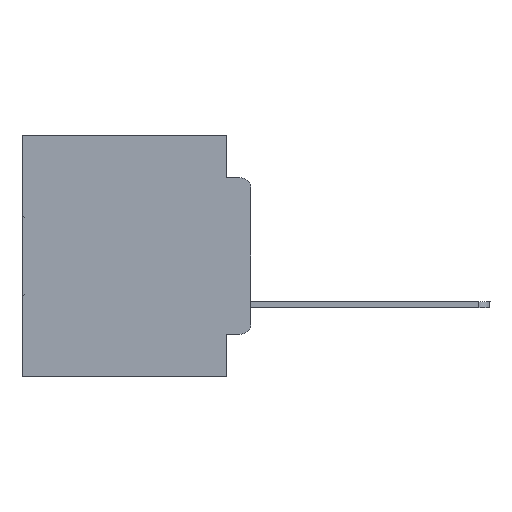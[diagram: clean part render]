
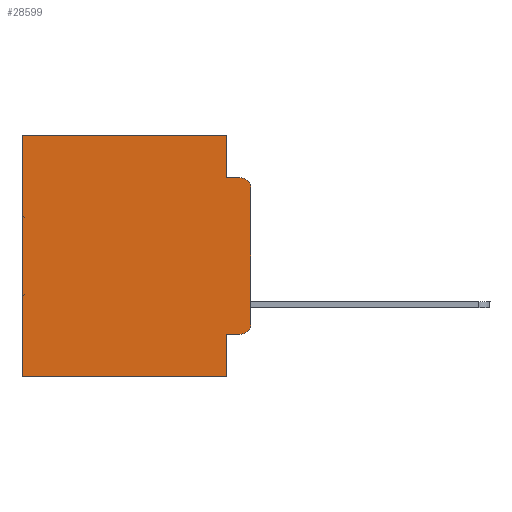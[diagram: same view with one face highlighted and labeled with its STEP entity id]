
A CAD part, left-side view. The second image highlights one B-rep face of the part: STEP entity #28599.
In plain terms, the highlighted planar face has unit normal (-1, 0, 0).
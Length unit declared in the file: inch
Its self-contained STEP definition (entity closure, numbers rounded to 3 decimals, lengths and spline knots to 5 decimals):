
#5 = ORIENTED_EDGE ( 'NONE', *, *, #15468, .F. ) ;
#101 = CARTESIAN_POINT ( 'NONE',  ( 0.298, 0.02, -0.0885 ) ) ;
#528 = LINE ( 'NONE', #17842, #26596 ) ;
#1420 = CARTESIAN_POINT ( 'NONE',  ( 0.298, 0.02, -0.4115 ) ) ;
#1983 = DIRECTION ( 'NONE',  ( 0., 0., -1. ) ) ;
#2085 = FACE_OUTER_BOUND ( 'NONE', #14257, .T. ) ;
#2849 = VERTEX_POINT ( 'NONE', #1420 ) ;
#3419 = VECTOR ( 'NONE', #27506, 39.37008 ) ;
#4102 = ORIENTED_EDGE ( 'NONE', *, *, #33243, .T. ) ;
#4320 = CARTESIAN_POINT ( 'NONE',  ( 0.298, 0.051, 0. ) ) ;
#4804 = ORIENTED_EDGE ( 'NONE', *, *, #7955, .F. ) ;
#5228 = PLANE ( 'NONE',  #32939 ) ;
#5334 = DIRECTION ( 'NONE',  ( 1., 0., 0. ) ) ;
#6238 = ORIENTED_EDGE ( 'NONE', *, *, #32335, .F. ) ;
#6807 = VECTOR ( 'NONE', #12660, 39.37008 ) ;
#7135 = VERTEX_POINT ( 'NONE', #10392 ) ;
#7210 = CARTESIAN_POINT ( 'NONE',  ( 0.298, 0.473, 0. ) ) ;
#7582 = AXIS2_PLACEMENT_3D ( 'NONE', #8883, #24767, #11425 ) ;
#7955 = EDGE_CURVE ( 'NONE', #19311, #17257, #26944, .T. ) ;
#8376 = LINE ( 'NONE', #23551, #8758 ) ;
#8644 = LINE ( 'NONE', #25972, #27678 ) ;
#8758 = VECTOR ( 'NONE', #10325, 39.37008 ) ;
#8883 = CARTESIAN_POINT ( 'NONE',  ( 0.298, 0.02, -0.3915 ) ) ;
#9470 = LINE ( 'NONE', #30316, #20276 ) ;
#9543 = CARTESIAN_POINT ( 'NONE',  ( 0.298, 0.051, -0.4115 ) ) ;
#10325 = DIRECTION ( 'NONE',  ( 0., -1., 0. ) ) ;
#10338 = ORIENTED_EDGE ( 'NONE', *, *, #34227, .F. ) ;
#10392 = CARTESIAN_POINT ( 'NONE',  ( 0.298, 0.051, -0.0885 ) ) ;
#10434 = CARTESIAN_POINT ( 'NONE',  ( 0.298, 0.051, -0.5 ) ) ;
#11283 = CIRCLE ( 'NONE', #25794, 0.02 ) ;
#11425 = DIRECTION ( 'NONE',  ( 0., 0., -1. ) ) ;
#12660 = DIRECTION ( 'NONE',  ( 0., 1., 0. ) ) ;
#12877 = DIRECTION ( 'NONE',  ( 0., 0., -1. ) ) ;
#13092 = DIRECTION ( 'NONE',  ( 0., 0., -1. ) ) ;
#13544 = EDGE_CURVE ( 'NONE', #22512, #19991, #24617, .T. ) ;
#14257 = EDGE_LOOP ( 'NONE', ( #6238, #22447, #5, #10338, #25697, #22107, #28660, #4804, #33003, #4102 ) ) ;
#14494 = CARTESIAN_POINT ( 'NONE',  ( 0.298, 0., 0. ) ) ;
#14996 = VERTEX_POINT ( 'NONE', #101 ) ;
#15468 = EDGE_CURVE ( 'NONE', #7135, #14996, #8376, .T. ) ;
#15526 = CARTESIAN_POINT ( 'NONE',  ( 0.298, 0.051, 0. ) ) ;
#15877 = CARTESIAN_POINT ( 'NONE',  ( 0.298, 0., 0. ) ) ;
#16544 = EDGE_CURVE ( 'NONE', #17257, #21843, #33093, .T. ) ;
#17202 = DIRECTION ( 'NONE',  ( 0., 0., -1. ) ) ;
#17257 = VERTEX_POINT ( 'NONE', #10434 ) ;
#17444 = CIRCLE ( 'NONE', #7582, 0.02 ) ;
#17842 = CARTESIAN_POINT ( 'NONE',  ( 0.298, 0.473, 0. ) ) ;
#18259 = VECTOR ( 'NONE', #23233, 39.37008 ) ;
#18435 = DIRECTION ( 'NONE',  ( 0., 0., -1. ) ) ;
#19311 = VERTEX_POINT ( 'NONE', #9543 ) ;
#19924 = VECTOR ( 'NONE', #13092, 39.37008 ) ;
#19991 = VERTEX_POINT ( 'NONE', #7210 ) ;
#20276 = VECTOR ( 'NONE', #30789, 39.37008 ) ;
#21843 = VERTEX_POINT ( 'NONE', #32787 ) ;
#22107 = ORIENTED_EDGE ( 'NONE', *, *, #27203, .T. ) ;
#22447 = ORIENTED_EDGE ( 'NONE', *, *, #23579, .T. ) ;
#22506 = CARTESIAN_POINT ( 'NONE',  ( 0.298, 0., -0.3915 ) ) ;
#22512 = VERTEX_POINT ( 'NONE', #4320 ) ;
#22669 = CARTESIAN_POINT ( 'NONE',  ( 0.298, 0., -0.5 ) ) ;
#23233 = DIRECTION ( 'NONE',  ( 0., 1., 0. ) ) ;
#23551 = CARTESIAN_POINT ( 'NONE',  ( 0.298, 0.051, -0.0885 ) ) ;
#23579 = EDGE_CURVE ( 'NONE', #33325, #14996, #11283, .T. ) ;
#24617 = LINE ( 'NONE', #26435, #6807 ) ;
#24767 = DIRECTION ( 'NONE',  ( -1., 0., 0. ) ) ;
#25280 = DIRECTION ( 'NONE',  ( -1., 0., 0. ) ) ;
#25504 = CARTESIAN_POINT ( 'NONE',  ( 0.298, 0.02, -0.1085 ) ) ;
#25697 = ORIENTED_EDGE ( 'NONE', *, *, #13544, .T. ) ;
#25794 = AXIS2_PLACEMENT_3D ( 'NONE', #25504, #25280, #17202 ) ;
#25972 = CARTESIAN_POINT ( 'NONE',  ( 0.298, 0.051, 0. ) ) ;
#26435 = CARTESIAN_POINT ( 'NONE',  ( 0.298, 0., 0. ) ) ;
#26596 = VECTOR ( 'NONE', #1983, 39.37008 ) ;
#26944 = LINE ( 'NONE', #15526, #19924 ) ;
#27203 = EDGE_CURVE ( 'NONE', #19991, #21843, #528, .T. ) ;
#27506 = DIRECTION ( 'NONE',  ( 0., 0., -1. ) ) ;
#27678 = VECTOR ( 'NONE', #12877, 39.37008 ) ;
#28599 = ADVANCED_FACE ( 'NONE', ( #2085 ), #5228, .F. ) ;
#28660 = ORIENTED_EDGE ( 'NONE', *, *, #16544, .F. ) ;
#30316 = CARTESIAN_POINT ( 'NONE',  ( 0.298, 0.051, -0.4115 ) ) ;
#30692 = VERTEX_POINT ( 'NONE', #22506 ) ;
#30695 = LINE ( 'NONE', #14494, #3419 ) ;
#30789 = DIRECTION ( 'NONE',  ( 0., -1., 0. ) ) ;
#32335 = EDGE_CURVE ( 'NONE', #33325, #30692, #30695, .T. ) ;
#32339 = CARTESIAN_POINT ( 'NONE',  ( 0.298, 0., -0.1085 ) ) ;
#32787 = CARTESIAN_POINT ( 'NONE',  ( 0.298, 0.473, -0.5 ) ) ;
#32939 = AXIS2_PLACEMENT_3D ( 'NONE', #15877, #5334, #18435 ) ;
#33003 = ORIENTED_EDGE ( 'NONE', *, *, #34117, .T. ) ;
#33093 = LINE ( 'NONE', #22669, #18259 ) ;
#33243 = EDGE_CURVE ( 'NONE', #2849, #30692, #17444, .T. ) ;
#33325 = VERTEX_POINT ( 'NONE', #32339 ) ;
#34117 = EDGE_CURVE ( 'NONE', #19311, #2849, #9470, .T. ) ;
#34227 = EDGE_CURVE ( 'NONE', #22512, #7135, #8644, .T. ) ;
